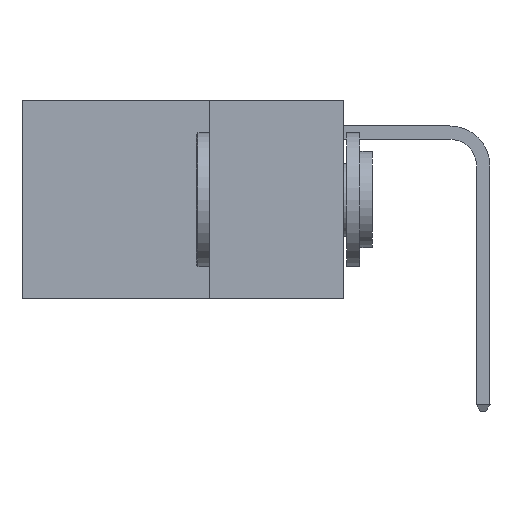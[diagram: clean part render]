
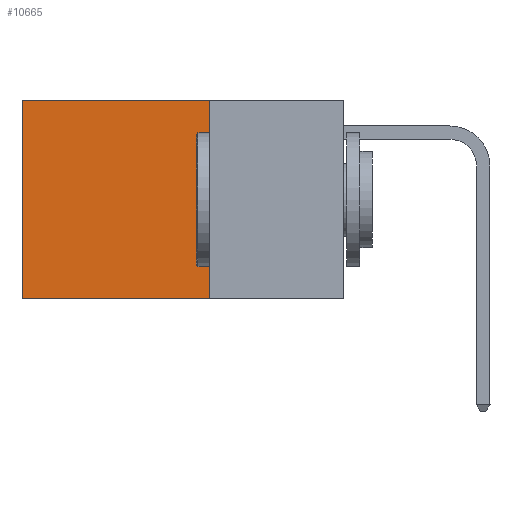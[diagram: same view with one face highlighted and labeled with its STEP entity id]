
A CAD part, left-side view. The second image highlights one B-rep face of the part: STEP entity #10665.
In plain terms, the highlighted planar face has unit normal (-1, 0, 0).
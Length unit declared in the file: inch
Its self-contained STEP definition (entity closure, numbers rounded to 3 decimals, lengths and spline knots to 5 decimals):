
#521 = CARTESIAN_POINT ( 'NONE',  ( 0.2625, 0.6, -0.37 ) ) ;
#558 = FACE_OUTER_BOUND ( 'NONE', #7991, .T. ) ;
#742 = LINE ( 'NONE', #15041, #12184 ) ;
#931 = DIRECTION ( 'NONE',  ( 0., 0., -1. ) ) ;
#1309 = DIRECTION ( 'NONE',  ( 0., 1., 0. ) ) ;
#1449 = DIRECTION ( 'NONE',  ( 0., 0., -1. ) ) ;
#2527 = ORIENTED_EDGE ( 'NONE', *, *, #18167, .F. ) ;
#3301 = VECTOR ( 'NONE', #17832, 39.37008 ) ;
#3391 = VERTEX_POINT ( 'NONE', #25821 ) ;
#4005 = LINE ( 'NONE', #10930, #3301 ) ;
#5550 = AXIS2_PLACEMENT_3D ( 'NONE', #28458, #14652, #931 ) ;
#7452 = EDGE_CURVE ( 'NONE', #3391, #20155, #742, .T. ) ;
#7634 = ORIENTED_EDGE ( 'NONE', *, *, #7452, .F. ) ;
#7991 = EDGE_LOOP ( 'NONE', ( #23069, #7634, #2527, #20016 ) ) ;
#9600 = CARTESIAN_POINT ( 'NONE',  ( 0.2625, 0.25, 0. ) ) ;
#10546 = CARTESIAN_POINT ( 'NONE',  ( 0.2625, 0.25, 0. ) ) ;
#10665 = ADVANCED_FACE ( 'NONE', ( #558 ), #12330, .F. ) ;
#10930 = CARTESIAN_POINT ( 'NONE',  ( 0.2625, 0.25, 0. ) ) ;
#12184 = VECTOR ( 'NONE', #1309, 39.37008 ) ;
#12330 = PLANE ( 'NONE',  #5550 ) ;
#13218 = CARTESIAN_POINT ( 'NONE',  ( 0.2625, 0.6, 0. ) ) ;
#14297 = EDGE_CURVE ( 'NONE', #20496, #20155, #17280, .T. ) ;
#14652 = DIRECTION ( 'NONE',  ( 1., 0., 0. ) ) ;
#15041 = CARTESIAN_POINT ( 'NONE',  ( 0.2625, 0.25, -0.37 ) ) ;
#17280 = LINE ( 'NONE', #21175, #28781 ) ;
#17832 = DIRECTION ( 'NONE',  ( 0., 1., 0. ) ) ;
#18167 = EDGE_CURVE ( 'NONE', #22132, #3391, #22509, .T. ) ;
#20016 = ORIENTED_EDGE ( 'NONE', *, *, #29441, .T. ) ;
#20155 = VERTEX_POINT ( 'NONE', #521 ) ;
#20496 = VERTEX_POINT ( 'NONE', #13218 ) ;
#21175 = CARTESIAN_POINT ( 'NONE',  ( 0.2625, 0.6, 0. ) ) ;
#21801 = VECTOR ( 'NONE', #1449, 39.37008 ) ;
#22132 = VERTEX_POINT ( 'NONE', #9600 ) ;
#22509 = LINE ( 'NONE', #10546, #21801 ) ;
#23069 = ORIENTED_EDGE ( 'NONE', *, *, #14297, .T. ) ;
#25821 = CARTESIAN_POINT ( 'NONE',  ( 0.2625, 0.25, -0.37 ) ) ;
#28073 = DIRECTION ( 'NONE',  ( 0., 0., -1. ) ) ;
#28458 = CARTESIAN_POINT ( 'NONE',  ( 0.2625, 0.25, 0. ) ) ;
#28781 = VECTOR ( 'NONE', #28073, 39.37008 ) ;
#29441 = EDGE_CURVE ( 'NONE', #22132, #20496, #4005, .T. ) ;
